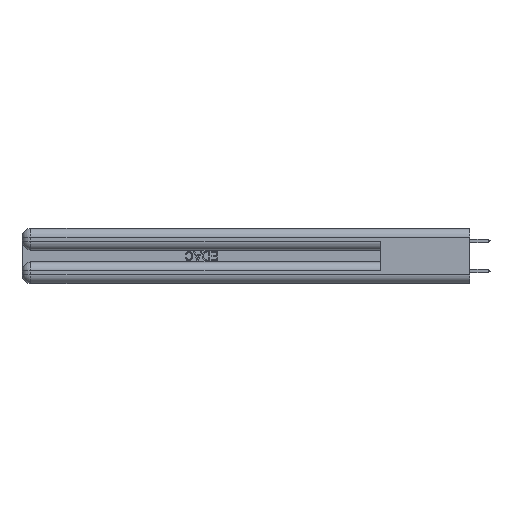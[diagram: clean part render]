
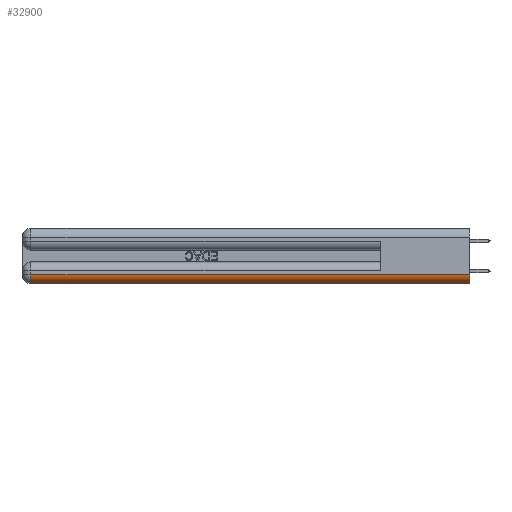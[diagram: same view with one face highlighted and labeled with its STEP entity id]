
A CAD part, left-side view. The second image highlights one B-rep face of the part: STEP entity #32900.
In plain terms, the highlighted cylindrical face has radius 1.524 mm (diameter 3.048 mm), a partial arc.
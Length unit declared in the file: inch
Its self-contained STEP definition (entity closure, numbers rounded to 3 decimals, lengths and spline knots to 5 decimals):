
#1380 = CARTESIAN_POINT ( 'NONE',  ( 0.06, 2.94, 0. ) ) ;
#2150 = CARTESIAN_POINT ( 'NONE',  ( 0.06, 0., 0.06 ) ) ;
#3485 = DIRECTION ( 'NONE',  ( 0., 1., 0. ) ) ;
#5329 = CARTESIAN_POINT ( 'NONE',  ( 0., 0., 0.06 ) ) ;
#5882 = CARTESIAN_POINT ( 'NONE',  ( 0.06, 0., 0.06 ) ) ;
#7122 = ORIENTED_EDGE ( 'NONE', *, *, #21306, .F. ) ;
#9365 = DIRECTION ( 'NONE',  ( 0., -1., 0. ) ) ;
#10905 = VERTEX_POINT ( 'NONE', #5329 ) ;
#10928 = EDGE_LOOP ( 'NONE', ( #28175, #29380, #26837, #7122 ) ) ;
#11577 = CIRCLE ( 'NONE', #43745, 0.06 ) ;
#12289 = VECTOR ( 'NONE', #37015, 39.37008 ) ;
#13393 = LINE ( 'NONE', #41318, #12289 ) ;
#13421 = AXIS2_PLACEMENT_3D ( 'NONE', #2150, #33716, #43987 ) ;
#13923 = VECTOR ( 'NONE', #14291, 39.37008 ) ;
#14213 = CARTESIAN_POINT ( 'NONE',  ( 0., 2.94, 0.06 ) ) ;
#14291 = DIRECTION ( 'NONE',  ( 0., 1., 0. ) ) ;
#19821 = VERTEX_POINT ( 'NONE', #25448 ) ;
#21306 = EDGE_CURVE ( 'NONE', #19821, #25194, #34224, .T. ) ;
#25041 = CYLINDRICAL_SURFACE ( 'NONE', #13421, 0.06 ) ;
#25109 = CARTESIAN_POINT ( 'NONE',  ( 0.06, 3., 0. ) ) ;
#25194 = VERTEX_POINT ( 'NONE', #1380 ) ;
#25448 = CARTESIAN_POINT ( 'NONE',  ( 0.06, 0., 0. ) ) ;
#26837 = ORIENTED_EDGE ( 'NONE', *, *, #38176, .F. ) ;
#27174 = AXIS2_PLACEMENT_3D ( 'NONE', #5882, #9365, #37163 ) ;
#28175 = ORIENTED_EDGE ( 'NONE', *, *, #43457, .F. ) ;
#28890 = FACE_OUTER_BOUND ( 'NONE', #10928, .T. ) ;
#29380 = ORIENTED_EDGE ( 'NONE', *, *, #43313, .F. ) ;
#32900 = ADVANCED_FACE ( 'NONE', ( #28890 ), #25041, .T. ) ;
#33716 = DIRECTION ( 'NONE',  ( 0., 1., 0. ) ) ;
#34224 = LINE ( 'NONE', #25109, #13923 ) ;
#37015 = DIRECTION ( 'NONE',  ( 0., -1., 0. ) ) ;
#37163 = DIRECTION ( 'NONE',  ( 0., 0., 1. ) ) ;
#38160 = CARTESIAN_POINT ( 'NONE',  ( 0.06, 2.94, 0.06 ) ) ;
#38176 = EDGE_CURVE ( 'NONE', #25194, #38333, #11577, .T. ) ;
#38233 = CIRCLE ( 'NONE', #27174, 0.06 ) ;
#38333 = VERTEX_POINT ( 'NONE', #14213 ) ;
#38597 = DIRECTION ( 'NONE',  ( 0., 0., 1. ) ) ;
#41318 = CARTESIAN_POINT ( 'NONE',  ( 0., 0., 0.06 ) ) ;
#43313 = EDGE_CURVE ( 'NONE', #38333, #10905, #13393, .T. ) ;
#43457 = EDGE_CURVE ( 'NONE', #10905, #19821, #38233, .T. ) ;
#43745 = AXIS2_PLACEMENT_3D ( 'NONE', #38160, #3485, #38597 ) ;
#43987 = DIRECTION ( 'NONE',  ( 0., 0., 1. ) ) ;
